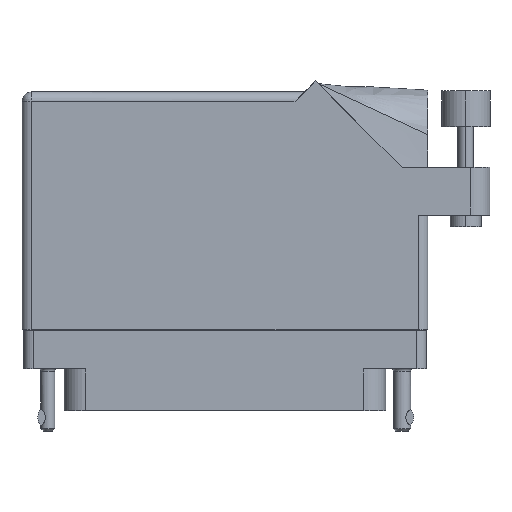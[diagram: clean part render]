
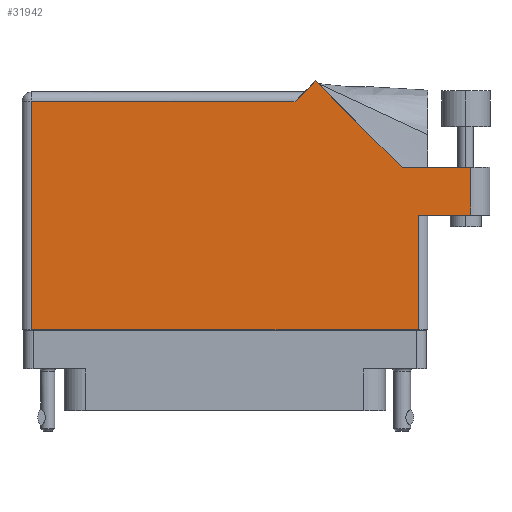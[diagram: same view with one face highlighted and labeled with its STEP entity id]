
A CAD part, front view. The second image highlights one B-rep face of the part: STEP entity #31942.
In plain terms, the highlighted face is planar.
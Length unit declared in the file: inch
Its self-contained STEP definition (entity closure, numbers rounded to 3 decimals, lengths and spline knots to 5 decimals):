
#20 = DIRECTION ( 'NONE',  ( 1., 0., 0. ) ) ;
#176 = DIRECTION ( 'NONE',  ( -1., 0., 0. ) ) ;
#2393 = ORIENTED_EDGE ( 'NONE', *, *, #17394, .T. ) ;
#3001 = CARTESIAN_POINT ( 'NONE',  ( 1.581, 0.944, 0.455 ) ) ;
#4908 = LINE ( 'NONE', #23571, #18948 ) ;
#5755 = VERTEX_POINT ( 'NONE', #45915 ) ;
#6346 = EDGE_CURVE ( 'NONE', #17435, #13758, #15085, .T. ) ;
#6567 = DIRECTION ( 'NONE',  ( -1., 0., 0. ) ) ;
#6938 = FACE_OUTER_BOUND ( 'NONE', #56717, .T. ) ;
#7278 = ORIENTED_EDGE ( 'NONE', *, *, #29959, .T. ) ;
#8227 = CARTESIAN_POINT ( 'NONE',  ( 1.244, -0.1, 0.455 ) ) ;
#9110 = VECTOR ( 'NONE', #55129, 39.37008 ) ;
#9201 = CARTESIAN_POINT ( 'NONE',  ( 1.14042, 0.944, 0.455 ) ) ;
#9772 = ORIENTED_EDGE ( 'NONE', *, *, #40822, .T. ) ;
#9879 = PLANE ( 'NONE',  #22538 ) ;
#9928 = ORIENTED_EDGE ( 'NONE', *, *, #54294, .T. ) ;
#11946 = DIRECTION ( 'NONE',  ( -1., 0., 0. ) ) ;
#12310 = DIRECTION ( 'NONE',  ( -0.707, 0.707, 0. ) ) ;
#12600 = CARTESIAN_POINT ( 'NONE',  ( 0.513, 1.43, 0.455 ) ) ;
#13758 = VERTEX_POINT ( 'NONE', #56506 ) ;
#14148 = VECTOR ( 'NONE', #11946, 39.37008 ) ;
#15085 = LINE ( 'NONE', #27101, #9110 ) ;
#17270 = CARTESIAN_POINT ( 'NONE',  ( 1.14042, 0.944, 0.455 ) ) ;
#17394 = EDGE_CURVE ( 'NONE', #37476, #47120, #20821, .T. ) ;
#17435 = VERTEX_POINT ( 'NONE', #8227 ) ;
#17513 = CARTESIAN_POINT ( 'NONE',  ( 1.581, 0.637, 0.455 ) ) ;
#17594 = VERTEX_POINT ( 'NONE', #17513 ) ;
#18601 = DIRECTION ( 'NONE',  ( 0., 0., -1. ) ) ;
#18948 = VECTOR ( 'NONE', #20, 39.37008 ) ;
#19937 = ORIENTED_EDGE ( 'NONE', *, *, #6346, .T. ) ;
#20821 = LINE ( 'NONE', #12600, #44430 ) ;
#22036 = CARTESIAN_POINT ( 'NONE',  ( 0.451, 1.368, 0.455 ) ) ;
#22538 = AXIS2_PLACEMENT_3D ( 'NONE', #42972, #18601, #176 ) ;
#23519 = VECTOR ( 'NONE', #12310, 39.37008 ) ;
#23571 = CARTESIAN_POINT ( 'NONE',  ( 1.306, 0.637, 0.455 ) ) ;
#26754 = DIRECTION ( 'NONE',  ( 0., 1., 0. ) ) ;
#26943 = VERTEX_POINT ( 'NONE', #60604 ) ;
#26984 = ORIENTED_EDGE ( 'NONE', *, *, #51230, .T. ) ;
#27101 = CARTESIAN_POINT ( 'NONE',  ( 1.244, 0.637, 0.455 ) ) ;
#27465 = LINE ( 'NONE', #39058, #41544 ) ;
#28544 = VERTEX_POINT ( 'NONE', #32277 ) ;
#29161 = VECTOR ( 'NONE', #46121, 39.37008 ) ;
#29628 = ORIENTED_EDGE ( 'NONE', *, *, #50368, .T. ) ;
#29959 = EDGE_CURVE ( 'NONE', #47120, #5755, #51021, .T. ) ;
#31666 = CARTESIAN_POINT ( 'NONE',  ( -1.244, -0.1, 0.455 ) ) ;
#31942 = ADVANCED_FACE ( 'NONE', ( #6938 ), #9879, .F. ) ;
#32048 = VECTOR ( 'NONE', #26754, 39.37008 ) ;
#32243 = DIRECTION ( 'NONE',  ( 0., -1., 0. ) ) ;
#32277 = CARTESIAN_POINT ( 'NONE',  ( 1.581, 0.944, 0.455 ) ) ;
#34001 = EDGE_CURVE ( 'NONE', #28544, #39596, #27465, .T. ) ;
#37476 = VERTEX_POINT ( 'NONE', #44476 ) ;
#39058 = CARTESIAN_POINT ( 'NONE',  ( 1.706, 0.944, 0.455 ) ) ;
#39596 = VERTEX_POINT ( 'NONE', #9201 ) ;
#40257 = CARTESIAN_POINT ( 'NONE',  ( -1.306, 1.368, 0.455 ) ) ;
#40822 = EDGE_CURVE ( 'NONE', #39596, #37476, #46416, .T. ) ;
#41544 = VECTOR ( 'NONE', #6567, 39.37008 ) ;
#42972 = CARTESIAN_POINT ( 'NONE',  ( -1.306, 1.43, 0.455 ) ) ;
#43212 = VECTOR ( 'NONE', #32243, 39.37008 ) ;
#44430 = VECTOR ( 'NONE', #45586, 39.37008 ) ;
#44476 = CARTESIAN_POINT ( 'NONE',  ( 0.58371, 1.50071, 0.455 ) ) ;
#44615 = LINE ( 'NONE', #3001, #32048 ) ;
#45344 = LINE ( 'NONE', #50245, #29161 ) ;
#45586 = DIRECTION ( 'NONE',  ( -0.707, -0.707, 0. ) ) ;
#45915 = CARTESIAN_POINT ( 'NONE',  ( -1.244, 1.368, 0.455 ) ) ;
#46121 = DIRECTION ( 'NONE',  ( 1., 0., 0. ) ) ;
#46416 = LINE ( 'NONE', #17270, #23519 ) ;
#47063 = ORIENTED_EDGE ( 'NONE', *, *, #53601, .T. ) ;
#47120 = VERTEX_POINT ( 'NONE', #22036 ) ;
#50245 = CARTESIAN_POINT ( 'NONE',  ( -1.306, -0.1, 0.455 ) ) ;
#50368 = EDGE_CURVE ( 'NONE', #26943, #17435, #45344, .T. ) ;
#51021 = LINE ( 'NONE', #40257, #14148 ) ;
#51230 = EDGE_CURVE ( 'NONE', #5755, #26943, #55647, .T. ) ;
#53601 = EDGE_CURVE ( 'NONE', #13758, #17594, #4908, .T. ) ;
#54294 = EDGE_CURVE ( 'NONE', #17594, #28544, #44615, .T. ) ;
#55129 = DIRECTION ( 'NONE',  ( 0., 1., 0. ) ) ;
#55647 = LINE ( 'NONE', #31666, #43212 ) ;
#56506 = CARTESIAN_POINT ( 'NONE',  ( 1.244, 0.637, 0.455 ) ) ;
#56717 = EDGE_LOOP ( 'NONE', ( #47063, #9928, #60276, #9772, #2393, #7278, #26984, #29628, #19937 ) ) ;
#60276 = ORIENTED_EDGE ( 'NONE', *, *, #34001, .T. ) ;
#60604 = CARTESIAN_POINT ( 'NONE',  ( -1.244, -0.1, 0.455 ) ) ;
